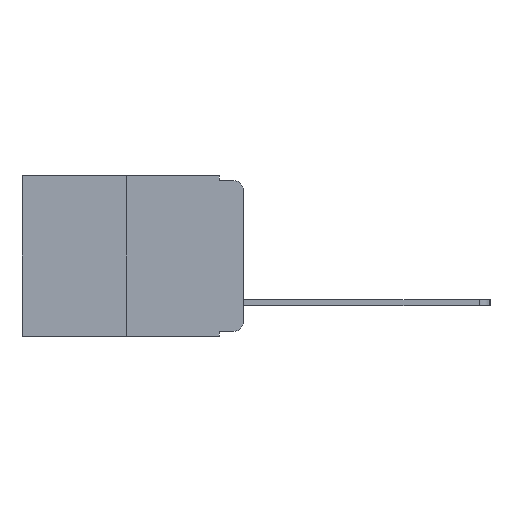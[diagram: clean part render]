
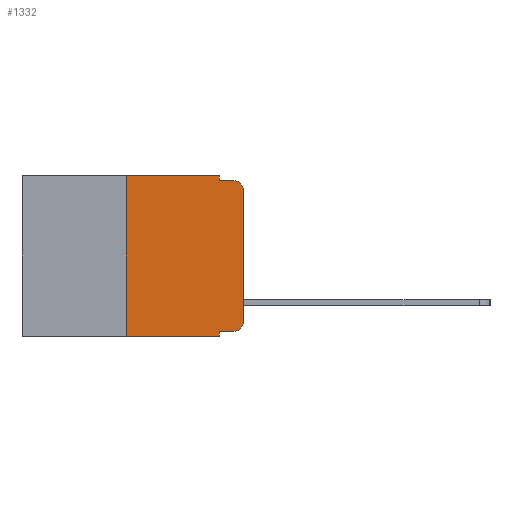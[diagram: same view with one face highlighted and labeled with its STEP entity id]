
A CAD part, left-side view. The second image highlights one B-rep face of the part: STEP entity #1332.
In plain terms, the highlighted planar face has unit normal (-1, 0, 0).
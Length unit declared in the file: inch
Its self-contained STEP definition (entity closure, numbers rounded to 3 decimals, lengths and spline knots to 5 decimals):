
#223 = DIRECTION ( 'NONE',  ( -1., 0., 0. ) ) ;
#349 = CARTESIAN_POINT ( 'NONE',  ( 0., 0.02, -0.03 ) ) ;
#410 = DIRECTION ( 'NONE',  ( 0., 0., -1. ) ) ;
#676 = VECTOR ( 'NONE', #10660, 39.37008 ) ;
#773 = FACE_OUTER_BOUND ( 'NONE', #17288, .T. ) ;
#823 = CARTESIAN_POINT ( 'NONE',  ( 0., 0.051, -0.333 ) ) ;
#986 = EDGE_CURVE ( 'NONE', #7912, #9499, #16909, .T. ) ;
#1242 = CARTESIAN_POINT ( 'NONE',  ( 0., 0.473, 0. ) ) ;
#1332 = ADVANCED_FACE ( 'NONE', ( #773 ), #4316, .F. ) ;
#1589 = DIRECTION ( 'NONE',  ( 0., 0., -1. ) ) ;
#1790 = LINE ( 'NONE', #14382, #5194 ) ;
#2158 = VERTEX_POINT ( 'NONE', #17430 ) ;
#2176 = VERTEX_POINT ( 'NONE', #12919 ) ;
#2263 = CARTESIAN_POINT ( 'NONE',  ( 0., 0.051, 0. ) ) ;
#2548 = EDGE_CURVE ( 'NONE', #15787, #2158, #14798, .T. ) ;
#2704 = DIRECTION ( 'NONE',  ( 0., -1., 0. ) ) ;
#2780 = ORIENTED_EDGE ( 'NONE', *, *, #4930, .T. ) ;
#3220 = CARTESIAN_POINT ( 'NONE',  ( 0., 0.25, -0.343 ) ) ;
#4285 = VECTOR ( 'NONE', #10936, 39.37008 ) ;
#4316 = PLANE ( 'NONE',  #10800 ) ;
#4529 = LINE ( 'NONE', #2263, #676 ) ;
#4678 = CIRCLE ( 'NONE', #9726, 0.02 ) ;
#4930 = EDGE_CURVE ( 'NONE', #7975, #15787, #1790, .T. ) ;
#5194 = VECTOR ( 'NONE', #17024, 39.37008 ) ;
#5419 = CARTESIAN_POINT ( 'NONE',  ( 0., 0.051, -0.343 ) ) ;
#5447 = EDGE_CURVE ( 'NONE', #12363, #2158, #15535, .T. ) ;
#6105 = CARTESIAN_POINT ( 'NONE',  ( 0., 0.25, 0. ) ) ;
#6205 = VECTOR ( 'NONE', #9878, 39.37008 ) ;
#6452 = DIRECTION ( 'NONE',  ( 0., -1., 0. ) ) ;
#6603 = VECTOR ( 'NONE', #14039, 39.37008 ) ;
#7368 = DIRECTION ( 'NONE',  ( 0., -1., 0. ) ) ;
#7417 = VERTEX_POINT ( 'NONE', #15800 ) ;
#7608 = EDGE_CURVE ( 'NONE', #10468, #9499, #4529, .T. ) ;
#7912 = VERTEX_POINT ( 'NONE', #3220 ) ;
#7933 = VECTOR ( 'NONE', #2704, 39.37008 ) ;
#7975 = VERTEX_POINT ( 'NONE', #8960 ) ;
#8292 = EDGE_CURVE ( 'NONE', #2176, #12363, #15547, .T. ) ;
#8297 = CARTESIAN_POINT ( 'NONE',  ( 0., 0.02, -0.313 ) ) ;
#8382 = ORIENTED_EDGE ( 'NONE', *, *, #8292, .F. ) ;
#8494 = VECTOR ( 'NONE', #7368, 39.37008 ) ;
#8960 = CARTESIAN_POINT ( 'NONE',  ( 0., 0., -0.313 ) ) ;
#8990 = ORIENTED_EDGE ( 'NONE', *, *, #5447, .F. ) ;
#9114 = DIRECTION ( 'NONE',  ( 1., 0., 0. ) ) ;
#9404 = ORIENTED_EDGE ( 'NONE', *, *, #14536, .T. ) ;
#9499 = VERTEX_POINT ( 'NONE', #5419 ) ;
#9603 = CARTESIAN_POINT ( 'NONE',  ( 0., 0.051, 0. ) ) ;
#9655 = DIRECTION ( 'NONE',  ( 0., 0., -1. ) ) ;
#9726 = AXIS2_PLACEMENT_3D ( 'NONE', #8297, #17578, #9655 ) ;
#9878 = DIRECTION ( 'NONE',  ( 0., -1., 0. ) ) ;
#9925 = CARTESIAN_POINT ( 'NONE',  ( 0., 0.473, -0.343 ) ) ;
#10086 = LINE ( 'NONE', #13214, #12366 ) ;
#10468 = VERTEX_POINT ( 'NONE', #823 ) ;
#10660 = DIRECTION ( 'NONE',  ( 0., 0., -1. ) ) ;
#10800 = AXIS2_PLACEMENT_3D ( 'NONE', #11993, #9114, #1589 ) ;
#10928 = CARTESIAN_POINT ( 'NONE',  ( 0., 0.051, -0.01 ) ) ;
#10936 = DIRECTION ( 'NONE',  ( 0., 0., -1. ) ) ;
#11419 = CARTESIAN_POINT ( 'NONE',  ( 0., 0.051, -0.01 ) ) ;
#11483 = ORIENTED_EDGE ( 'NONE', *, *, #986, .T. ) ;
#11907 = LINE ( 'NONE', #1242, #7933 ) ;
#11993 = CARTESIAN_POINT ( 'NONE',  ( 0., 0.473, 0. ) ) ;
#12363 = VERTEX_POINT ( 'NONE', #10928 ) ;
#12366 = VECTOR ( 'NONE', #6452, 39.37008 ) ;
#12715 = CARTESIAN_POINT ( 'NONE',  ( 0., 0.25, 0. ) ) ;
#12919 = CARTESIAN_POINT ( 'NONE',  ( 0., 0.051, 0. ) ) ;
#12952 = ORIENTED_EDGE ( 'NONE', *, *, #16320, .T. ) ;
#13214 = CARTESIAN_POINT ( 'NONE',  ( 0., 0.051, -0.333 ) ) ;
#13378 = ORIENTED_EDGE ( 'NONE', *, *, #7608, .F. ) ;
#14039 = DIRECTION ( 'NONE',  ( 0., 0., 1. ) ) ;
#14382 = CARTESIAN_POINT ( 'NONE',  ( 0., 0., 0. ) ) ;
#14536 = EDGE_CURVE ( 'NONE', #7417, #7975, #4678, .T. ) ;
#14623 = ORIENTED_EDGE ( 'NONE', *, *, #17158, .F. ) ;
#14788 = AXIS2_PLACEMENT_3D ( 'NONE', #349, #223, #410 ) ;
#14798 = CIRCLE ( 'NONE', #14788, 0.02 ) ;
#15006 = ORIENTED_EDGE ( 'NONE', *, *, #17273, .F. ) ;
#15535 = LINE ( 'NONE', #11419, #8494 ) ;
#15547 = LINE ( 'NONE', #9603, #4285 ) ;
#15787 = VERTEX_POINT ( 'NONE', #17475 ) ;
#15800 = CARTESIAN_POINT ( 'NONE',  ( 0., 0.02, -0.333 ) ) ;
#16320 = EDGE_CURVE ( 'NONE', #10468, #7417, #10086, .T. ) ;
#16455 = ORIENTED_EDGE ( 'NONE', *, *, #2548, .T. ) ;
#16786 = VERTEX_POINT ( 'NONE', #6105 ) ;
#16846 = LINE ( 'NONE', #12715, #6603 ) ;
#16909 = LINE ( 'NONE', #9925, #6205 ) ;
#17024 = DIRECTION ( 'NONE',  ( 0., 0., 1. ) ) ;
#17158 = EDGE_CURVE ( 'NONE', #16786, #2176, #11907, .T. ) ;
#17273 = EDGE_CURVE ( 'NONE', #7912, #16786, #16846, .T. ) ;
#17288 = EDGE_LOOP ( 'NONE', ( #2780, #16455, #8990, #8382, #14623, #15006, #11483, #13378, #12952, #9404 ) ) ;
#17430 = CARTESIAN_POINT ( 'NONE',  ( 0., 0.02, -0.01 ) ) ;
#17475 = CARTESIAN_POINT ( 'NONE',  ( 0., 0., -0.03 ) ) ;
#17578 = DIRECTION ( 'NONE',  ( -1., 0., 0. ) ) ;
